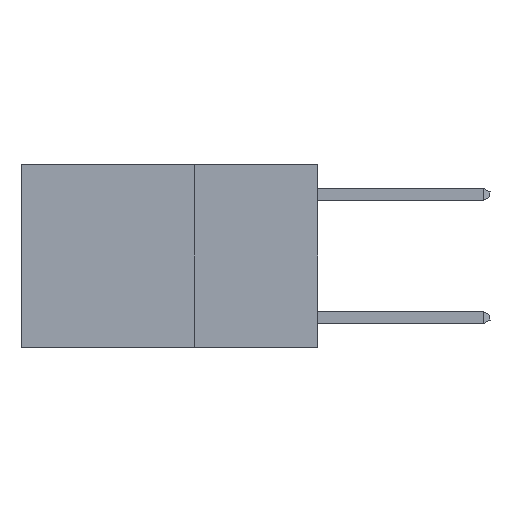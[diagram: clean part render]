
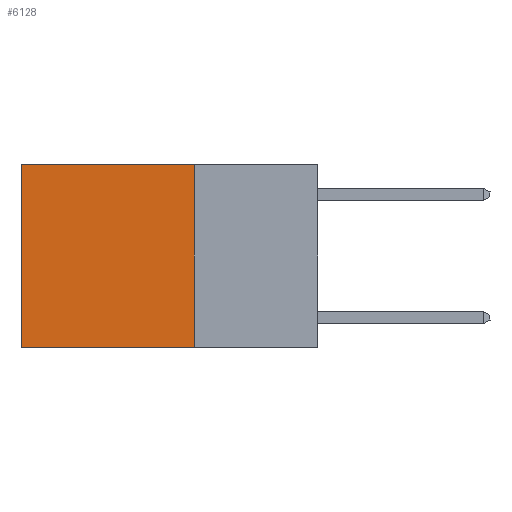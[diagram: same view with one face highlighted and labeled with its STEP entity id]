
A CAD part, left-side view. The second image highlights one B-rep face of the part: STEP entity #6128.
In plain terms, the highlighted planar face has unit normal (-1, 0, 0).
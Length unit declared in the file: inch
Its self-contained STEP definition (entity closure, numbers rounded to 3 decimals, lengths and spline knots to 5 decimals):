
#122 = DIRECTION ( 'NONE',  ( 0., 1., 0. ) ) ;
#218 = CARTESIAN_POINT ( 'NONE',  ( 0.2625, 0.25, -0.37 ) ) ;
#676 = ORIENTED_EDGE ( 'NONE', *, *, #9855, .T. ) ;
#886 = VERTEX_POINT ( 'NONE', #17190 ) ;
#934 = VECTOR ( 'NONE', #122, 39.37008 ) ;
#1464 = LINE ( 'NONE', #12266, #2253 ) ;
#2253 = VECTOR ( 'NONE', #18532, 39.37008 ) ;
#2426 = CARTESIAN_POINT ( 'NONE',  ( 0.2625, 0.25, 0. ) ) ;
#3752 = VECTOR ( 'NONE', #5611, 39.37008 ) ;
#5191 = ORIENTED_EDGE ( 'NONE', *, *, #16621, .F. ) ;
#5611 = DIRECTION ( 'NONE',  ( 0., 1., 0. ) ) ;
#5820 = VECTOR ( 'NONE', #12752, 39.37008 ) ;
#6128 = ADVANCED_FACE ( 'NONE', ( #19540 ), #8899, .F. ) ;
#6162 = EDGE_CURVE ( 'NONE', #17942, #11019, #18307, .T. ) ;
#8690 = DIRECTION ( 'NONE',  ( 1., 0., 0. ) ) ;
#8899 = PLANE ( 'NONE',  #15757 ) ;
#8993 = DIRECTION ( 'NONE',  ( 0., 0., -1. ) ) ;
#9855 = EDGE_CURVE ( 'NONE', #11019, #886, #1464, .T. ) ;
#10206 = CARTESIAN_POINT ( 'NONE',  ( 0.2625, 0.25, -0.37 ) ) ;
#10956 = LINE ( 'NONE', #17087, #5820 ) ;
#11019 = VERTEX_POINT ( 'NONE', #18030 ) ;
#12266 = CARTESIAN_POINT ( 'NONE',  ( 0.2625, 0.6, 0. ) ) ;
#12337 = EDGE_CURVE ( 'NONE', #17942, #19781, #10956, .T. ) ;
#12752 = DIRECTION ( 'NONE',  ( 0., 0., -1. ) ) ;
#14185 = LINE ( 'NONE', #218, #934 ) ;
#15757 = AXIS2_PLACEMENT_3D ( 'NONE', #18005, #8690, #8993 ) ;
#16195 = ORIENTED_EDGE ( 'NONE', *, *, #12337, .F. ) ;
#16229 = ORIENTED_EDGE ( 'NONE', *, *, #6162, .T. ) ;
#16621 = EDGE_CURVE ( 'NONE', #19781, #886, #14185, .T. ) ;
#17087 = CARTESIAN_POINT ( 'NONE',  ( 0.2625, 0.25, 0. ) ) ;
#17190 = CARTESIAN_POINT ( 'NONE',  ( 0.2625, 0.6, -0.37 ) ) ;
#17942 = VERTEX_POINT ( 'NONE', #2426 ) ;
#18005 = CARTESIAN_POINT ( 'NONE',  ( 0.2625, 0.25, 0. ) ) ;
#18030 = CARTESIAN_POINT ( 'NONE',  ( 0.2625, 0.6, 0. ) ) ;
#18307 = LINE ( 'NONE', #19749, #3752 ) ;
#18532 = DIRECTION ( 'NONE',  ( 0., 0., -1. ) ) ;
#19272 = EDGE_LOOP ( 'NONE', ( #676, #5191, #16195, #16229 ) ) ;
#19540 = FACE_OUTER_BOUND ( 'NONE', #19272, .T. ) ;
#19749 = CARTESIAN_POINT ( 'NONE',  ( 0.2625, 0.25, 0. ) ) ;
#19781 = VERTEX_POINT ( 'NONE', #10206 ) ;
